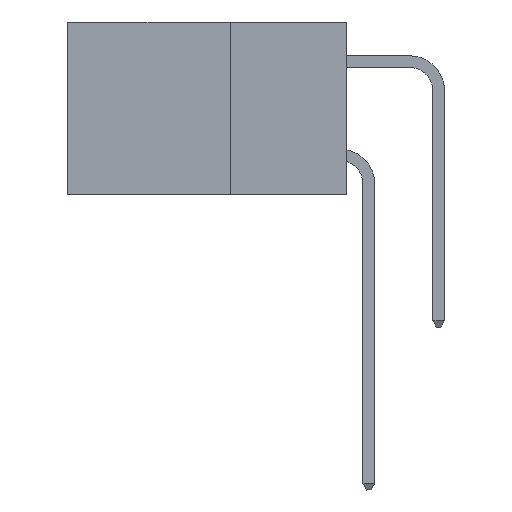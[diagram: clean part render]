
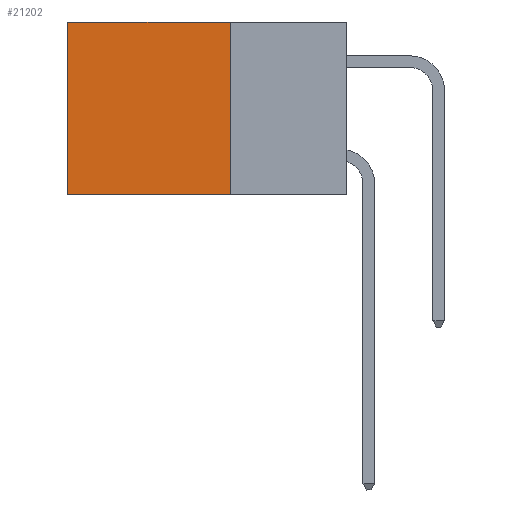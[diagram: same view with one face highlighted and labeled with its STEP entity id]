
A CAD part, left-side view. The second image highlights one B-rep face of the part: STEP entity #21202.
In plain terms, the highlighted planar face has unit normal (-1, 0, 0).
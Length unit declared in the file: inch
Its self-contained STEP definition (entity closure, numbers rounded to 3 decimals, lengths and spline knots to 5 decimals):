
#289 = VERTEX_POINT ( 'NONE', #4402 ) ;
#371 = ORIENTED_EDGE ( 'NONE', *, *, #5834, .T. ) ;
#477 = EDGE_CURVE ( 'NONE', #289, #2961, #12570, .T. ) ;
#601 = DIRECTION ( 'NONE',  ( 0., 1., 0. ) ) ;
#653 = CARTESIAN_POINT ( 'NONE',  ( 0.2875, 0.6, 0. ) ) ;
#792 = VERTEX_POINT ( 'NONE', #16091 ) ;
#1707 = CARTESIAN_POINT ( 'NONE',  ( 0.2875, 0.25, 0. ) ) ;
#2560 = ORIENTED_EDGE ( 'NONE', *, *, #15882, .F. ) ;
#2961 = VERTEX_POINT ( 'NONE', #20924 ) ;
#3394 = VECTOR ( 'NONE', #19159, 39.37008 ) ;
#3538 = PLANE ( 'NONE',  #22918 ) ;
#4121 = ORIENTED_EDGE ( 'NONE', *, *, #14883, .T. ) ;
#4402 = CARTESIAN_POINT ( 'NONE',  ( 0.2875, 0.25, 0. ) ) ;
#5514 = DIRECTION ( 'NONE',  ( 1., 0., 0. ) ) ;
#5834 = EDGE_CURVE ( 'NONE', #289, #13982, #9046, .T. ) ;
#7515 = VECTOR ( 'NONE', #10961, 39.37008 ) ;
#9046 = LINE ( 'NONE', #22877, #3394 ) ;
#10022 = CARTESIAN_POINT ( 'NONE',  ( 0.2875, 0.25, 0. ) ) ;
#10066 = CARTESIAN_POINT ( 'NONE',  ( 0.2875, 0.25, -0.37 ) ) ;
#10961 = DIRECTION ( 'NONE',  ( 0., 0., -1. ) ) ;
#12570 = LINE ( 'NONE', #10022, #7515 ) ;
#12752 = LINE ( 'NONE', #10066, #17248 ) ;
#13982 = VERTEX_POINT ( 'NONE', #24227 ) ;
#14883 = EDGE_CURVE ( 'NONE', #13982, #792, #20288, .T. ) ;
#15232 = VECTOR ( 'NONE', #23532, 39.37008 ) ;
#15882 = EDGE_CURVE ( 'NONE', #2961, #792, #12752, .T. ) ;
#16091 = CARTESIAN_POINT ( 'NONE',  ( 0.2875, 0.6, -0.37 ) ) ;
#17248 = VECTOR ( 'NONE', #601, 39.37008 ) ;
#18878 = DIRECTION ( 'NONE',  ( 0., 0., -1. ) ) ;
#19159 = DIRECTION ( 'NONE',  ( 0., 1., 0. ) ) ;
#19929 = ORIENTED_EDGE ( 'NONE', *, *, #477, .F. ) ;
#20288 = LINE ( 'NONE', #653, #15232 ) ;
#20924 = CARTESIAN_POINT ( 'NONE',  ( 0.2875, 0.25, -0.37 ) ) ;
#21202 = ADVANCED_FACE ( 'NONE', ( #24167 ), #3538, .F. ) ;
#22323 = EDGE_LOOP ( 'NONE', ( #4121, #2560, #19929, #371 ) ) ;
#22877 = CARTESIAN_POINT ( 'NONE',  ( 0.2875, 0.25, 0. ) ) ;
#22918 = AXIS2_PLACEMENT_3D ( 'NONE', #1707, #5514, #18878 ) ;
#23532 = DIRECTION ( 'NONE',  ( 0., 0., -1. ) ) ;
#24167 = FACE_OUTER_BOUND ( 'NONE', #22323, .T. ) ;
#24227 = CARTESIAN_POINT ( 'NONE',  ( 0.2875, 0.6, 0. ) ) ;
